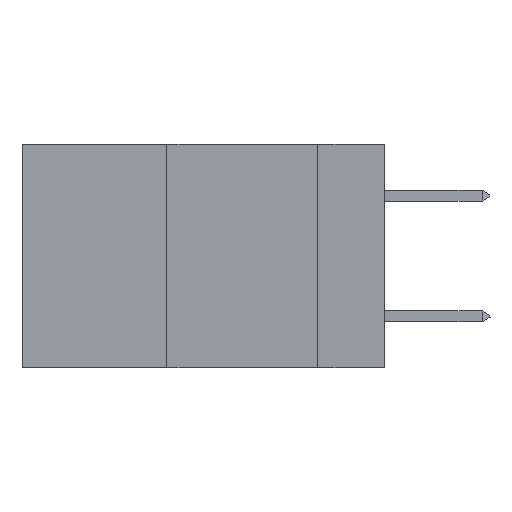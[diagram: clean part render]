
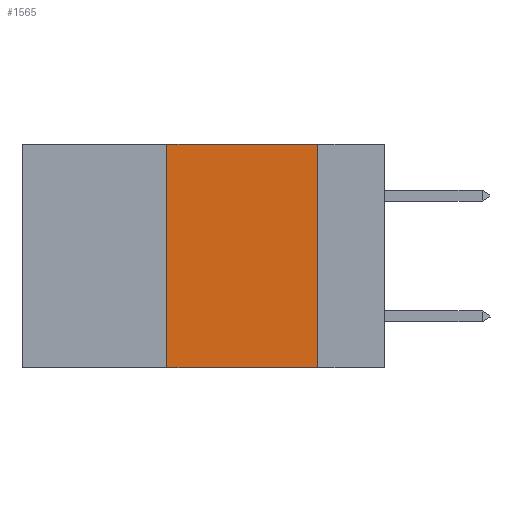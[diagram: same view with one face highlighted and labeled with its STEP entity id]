
A CAD part, left-side view. The second image highlights one B-rep face of the part: STEP entity #1565.
In plain terms, the highlighted planar face has unit normal (-1, 0, 0).
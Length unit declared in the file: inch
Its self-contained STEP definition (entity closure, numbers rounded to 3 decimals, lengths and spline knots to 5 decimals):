
#194 = AXIS2_PLACEMENT_3D ( 'NONE', #6140, #8860, #8952 ) ;
#211 = EDGE_CURVE ( 'NONE', #7614, #6099, #3115, .T. ) ;
#1202 = VECTOR ( 'NONE', #3269, 39.37008 ) ;
#1405 = CARTESIAN_POINT ( 'NONE',  ( 0., 0.11, 0. ) ) ;
#1487 = EDGE_CURVE ( 'NONE', #7614, #6335, #7822, .T. ) ;
#1565 = ADVANCED_FACE ( 'NONE', ( #8485 ), #8233, .F. ) ;
#1705 = DIRECTION ( 'NONE',  ( 0., -1., 0. ) ) ;
#1753 = VERTEX_POINT ( 'NONE', #1405 ) ;
#1808 = CARTESIAN_POINT ( 'NONE',  ( 0., 0.11, -0.37 ) ) ;
#1873 = EDGE_CURVE ( 'NONE', #1753, #6335, #2973, .T. ) ;
#2044 = ORIENTED_EDGE ( 'NONE', *, *, #1873, .F. ) ;
#2366 = CARTESIAN_POINT ( 'NONE',  ( 0., 0.36, 0. ) ) ;
#2378 = ORIENTED_EDGE ( 'NONE', *, *, #8445, .F. ) ;
#2472 = CARTESIAN_POINT ( 'NONE',  ( 0., 0.36, 0. ) ) ;
#2747 = VECTOR ( 'NONE', #5317, 39.37008 ) ;
#2973 = LINE ( 'NONE', #8642, #4426 ) ;
#3115 = LINE ( 'NONE', #2472, #1202 ) ;
#3269 = DIRECTION ( 'NONE',  ( 0., 0., 1. ) ) ;
#3616 = DIRECTION ( 'NONE',  ( 0., 0., -1. ) ) ;
#4426 = VECTOR ( 'NONE', #3616, 39.37008 ) ;
#4576 = VECTOR ( 'NONE', #1705, 39.37008 ) ;
#4622 = CARTESIAN_POINT ( 'NONE',  ( 0., 0.6, 0. ) ) ;
#4991 = CARTESIAN_POINT ( 'NONE',  ( 0., 0.36, -0.37 ) ) ;
#5317 = DIRECTION ( 'NONE',  ( 0., -1., 0. ) ) ;
#5342 = CARTESIAN_POINT ( 'NONE',  ( 0., 0.6, -0.37 ) ) ;
#6001 = EDGE_LOOP ( 'NONE', ( #2044, #2378, #6194, #8010 ) ) ;
#6099 = VERTEX_POINT ( 'NONE', #2366 ) ;
#6140 = CARTESIAN_POINT ( 'NONE',  ( 0., 0.6, 0. ) ) ;
#6194 = ORIENTED_EDGE ( 'NONE', *, *, #211, .F. ) ;
#6335 = VERTEX_POINT ( 'NONE', #1808 ) ;
#7329 = LINE ( 'NONE', #4622, #4576 ) ;
#7614 = VERTEX_POINT ( 'NONE', #4991 ) ;
#7822 = LINE ( 'NONE', #5342, #2747 ) ;
#8010 = ORIENTED_EDGE ( 'NONE', *, *, #1487, .T. ) ;
#8233 = PLANE ( 'NONE',  #194 ) ;
#8445 = EDGE_CURVE ( 'NONE', #6099, #1753, #7329, .T. ) ;
#8485 = FACE_OUTER_BOUND ( 'NONE', #6001, .T. ) ;
#8642 = CARTESIAN_POINT ( 'NONE',  ( 0., 0.11, 0. ) ) ;
#8860 = DIRECTION ( 'NONE',  ( 1., 0., 0. ) ) ;
#8952 = DIRECTION ( 'NONE',  ( 0., 0., -1. ) ) ;
